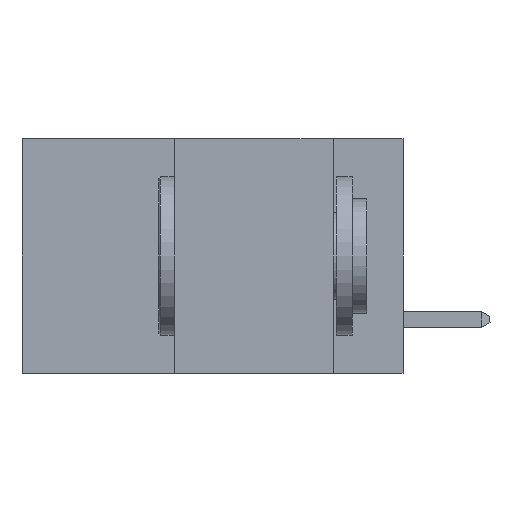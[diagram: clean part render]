
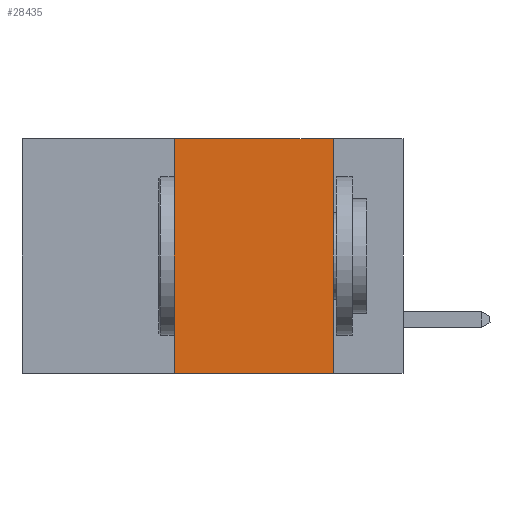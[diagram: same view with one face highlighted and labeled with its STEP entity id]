
A CAD part, left-side view. The second image highlights one B-rep face of the part: STEP entity #28435.
In plain terms, the highlighted planar face has unit normal (-1, 0, 0).
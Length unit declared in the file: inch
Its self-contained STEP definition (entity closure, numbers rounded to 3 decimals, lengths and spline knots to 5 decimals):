
#288 = VERTEX_POINT ( 'NONE', #19005 ) ;
#1751 = ORIENTED_EDGE ( 'NONE', *, *, #4345, .F. ) ;
#1795 = VERTEX_POINT ( 'NONE', #28167 ) ;
#2815 = PLANE ( 'NONE',  #5557 ) ;
#3540 = CARTESIAN_POINT ( 'NONE',  ( 0., 0.6, 0. ) ) ;
#4345 = EDGE_CURVE ( 'NONE', #29429, #288, #15508, .T. ) ;
#4556 = EDGE_LOOP ( 'NONE', ( #29530, #29868, #1751, #19600 ) ) ;
#5435 = LINE ( 'NONE', #3540, #29142 ) ;
#5557 = AXIS2_PLACEMENT_3D ( 'NONE', #28127, #21415, #7554 ) ;
#6091 = VERTEX_POINT ( 'NONE', #11581 ) ;
#7194 = VECTOR ( 'NONE', #12468, 39.37008 ) ;
#7554 = DIRECTION ( 'NONE',  ( 0., 0., -1. ) ) ;
#8670 = LINE ( 'NONE', #21507, #7194 ) ;
#9309 = VECTOR ( 'NONE', #18287, 39.37008 ) ;
#10974 = EDGE_CURVE ( 'NONE', #288, #6091, #5435, .T. ) ;
#11444 = CARTESIAN_POINT ( 'NONE',  ( 0., 0.36, 0. ) ) ;
#11581 = CARTESIAN_POINT ( 'NONE',  ( 0., 0.11, 0. ) ) ;
#11595 = VECTOR ( 'NONE', #23071, 39.37008 ) ;
#12038 = EDGE_CURVE ( 'NONE', #6091, #1795, #8670, .T. ) ;
#12332 = LINE ( 'NONE', #16197, #11595 ) ;
#12468 = DIRECTION ( 'NONE',  ( 0., 0., -1. ) ) ;
#13012 = DIRECTION ( 'NONE',  ( 0., -1., 0. ) ) ;
#15508 = LINE ( 'NONE', #11444, #9309 ) ;
#15800 = CARTESIAN_POINT ( 'NONE',  ( 0., 0.36, -0.37 ) ) ;
#16197 = CARTESIAN_POINT ( 'NONE',  ( 0., 0.6, -0.37 ) ) ;
#18067 = FACE_OUTER_BOUND ( 'NONE', #4556, .T. ) ;
#18287 = DIRECTION ( 'NONE',  ( 0., 0., 1. ) ) ;
#19005 = CARTESIAN_POINT ( 'NONE',  ( 0., 0.36, 0. ) ) ;
#19600 = ORIENTED_EDGE ( 'NONE', *, *, #19822, .T. ) ;
#19822 = EDGE_CURVE ( 'NONE', #29429, #1795, #12332, .T. ) ;
#21415 = DIRECTION ( 'NONE',  ( 1., 0., 0. ) ) ;
#21507 = CARTESIAN_POINT ( 'NONE',  ( 0., 0.11, 0. ) ) ;
#23071 = DIRECTION ( 'NONE',  ( 0., -1., 0. ) ) ;
#28127 = CARTESIAN_POINT ( 'NONE',  ( 0., 0.6, 0. ) ) ;
#28167 = CARTESIAN_POINT ( 'NONE',  ( 0., 0.11, -0.37 ) ) ;
#28435 = ADVANCED_FACE ( 'NONE', ( #18067 ), #2815, .F. ) ;
#29142 = VECTOR ( 'NONE', #13012, 39.37008 ) ;
#29429 = VERTEX_POINT ( 'NONE', #15800 ) ;
#29530 = ORIENTED_EDGE ( 'NONE', *, *, #12038, .F. ) ;
#29868 = ORIENTED_EDGE ( 'NONE', *, *, #10974, .F. ) ;
